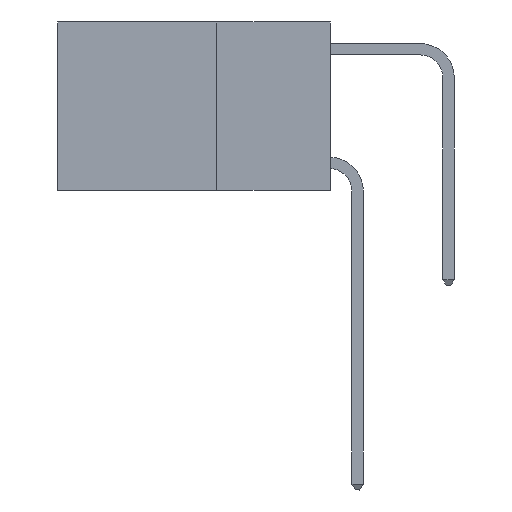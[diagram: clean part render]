
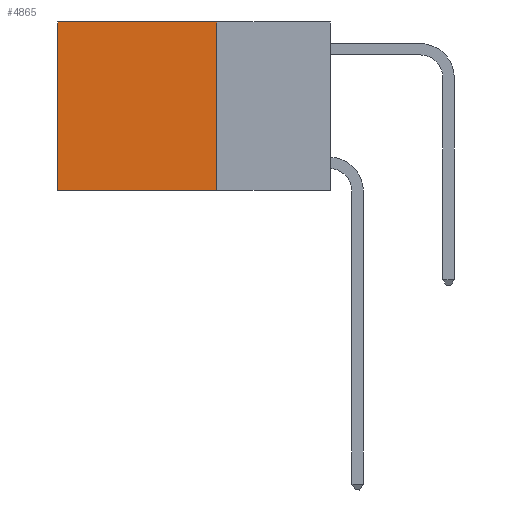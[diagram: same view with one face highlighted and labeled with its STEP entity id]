
A CAD part, left-side view. The second image highlights one B-rep face of the part: STEP entity #4865.
In plain terms, the highlighted planar face has unit normal (-1, 0, 0).
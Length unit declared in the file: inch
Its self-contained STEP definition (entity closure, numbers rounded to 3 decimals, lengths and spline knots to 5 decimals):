
#108 = EDGE_LOOP ( 'NONE', ( #15350, #15566, #1898, #8297 ) ) ;
#1898 = ORIENTED_EDGE ( 'NONE', *, *, #12476, .F. ) ;
#1972 = LINE ( 'NONE', #6319, #10021 ) ;
#2548 = CARTESIAN_POINT ( 'NONE',  ( 0.2625, 0.25, -0.37 ) ) ;
#2744 = CARTESIAN_POINT ( 'NONE',  ( 0.2625, 0.25, 0. ) ) ;
#2915 = EDGE_CURVE ( 'NONE', #6903, #14752, #18767, .T. ) ;
#3624 = VERTEX_POINT ( 'NONE', #9472 ) ;
#4280 = EDGE_CURVE ( 'NONE', #14208, #14752, #18961, .T. ) ;
#4345 = DIRECTION ( 'NONE',  ( 0., 0., -1. ) ) ;
#4865 = ADVANCED_FACE ( 'NONE', ( #16801 ), #12321, .F. ) ;
#5341 = AXIS2_PLACEMENT_3D ( 'NONE', #2744, #13928, #4345 ) ;
#6155 = CARTESIAN_POINT ( 'NONE',  ( 0.2625, 0.25, 0. ) ) ;
#6241 = DIRECTION ( 'NONE',  ( 0., 1., 0. ) ) ;
#6319 = CARTESIAN_POINT ( 'NONE',  ( 0.2625, 0.25, 0. ) ) ;
#6671 = EDGE_CURVE ( 'NONE', #3624, #6903, #1972, .T. ) ;
#6903 = VERTEX_POINT ( 'NONE', #13298 ) ;
#8297 = ORIENTED_EDGE ( 'NONE', *, *, #6671, .T. ) ;
#9091 = DIRECTION ( 'NONE',  ( 0., 0., -1. ) ) ;
#9472 = CARTESIAN_POINT ( 'NONE',  ( 0.2625, 0.25, 0. ) ) ;
#9512 = DIRECTION ( 'NONE',  ( 0., 1., 0. ) ) ;
#9901 = VECTOR ( 'NONE', #9091, 39.37008 ) ;
#10021 = VECTOR ( 'NONE', #9512, 39.37008 ) ;
#10159 = LINE ( 'NONE', #6155, #13900 ) ;
#10592 = VECTOR ( 'NONE', #6241, 39.37008 ) ;
#12321 = PLANE ( 'NONE',  #5341 ) ;
#12476 = EDGE_CURVE ( 'NONE', #3624, #14208, #10159, .T. ) ;
#13298 = CARTESIAN_POINT ( 'NONE',  ( 0.2625, 0.6, 0. ) ) ;
#13900 = VECTOR ( 'NONE', #18785, 39.37008 ) ;
#13928 = DIRECTION ( 'NONE',  ( 1., 0., 0. ) ) ;
#14151 = CARTESIAN_POINT ( 'NONE',  ( 0.2625, 0.25, -0.37 ) ) ;
#14208 = VERTEX_POINT ( 'NONE', #2548 ) ;
#14752 = VERTEX_POINT ( 'NONE', #16614 ) ;
#15350 = ORIENTED_EDGE ( 'NONE', *, *, #2915, .T. ) ;
#15566 = ORIENTED_EDGE ( 'NONE', *, *, #4280, .F. ) ;
#16614 = CARTESIAN_POINT ( 'NONE',  ( 0.2625, 0.6, -0.37 ) ) ;
#16801 = FACE_OUTER_BOUND ( 'NONE', #108, .T. ) ;
#18506 = CARTESIAN_POINT ( 'NONE',  ( 0.2625, 0.6, 0. ) ) ;
#18767 = LINE ( 'NONE', #18506, #9901 ) ;
#18785 = DIRECTION ( 'NONE',  ( 0., 0., -1. ) ) ;
#18961 = LINE ( 'NONE', #14151, #10592 ) ;
